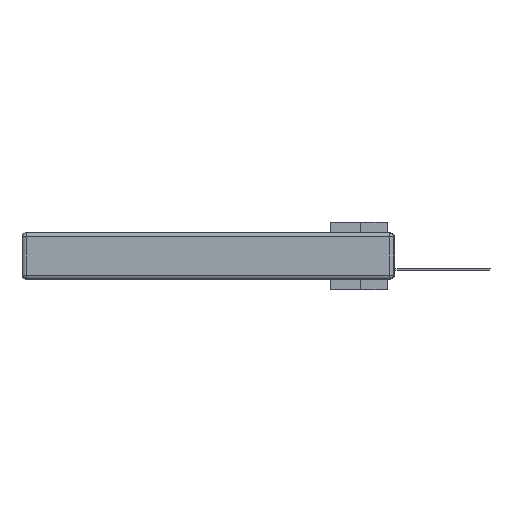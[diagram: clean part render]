
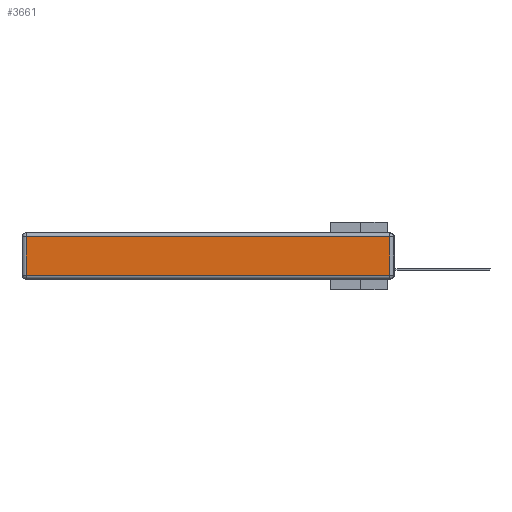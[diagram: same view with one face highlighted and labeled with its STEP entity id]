
A CAD part, left-side view. The second image highlights one B-rep face of the part: STEP entity #3661.
In plain terms, the highlighted planar face has unit normal (-1, 0, 0).
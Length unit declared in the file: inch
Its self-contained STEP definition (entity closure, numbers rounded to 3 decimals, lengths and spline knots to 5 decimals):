
#362 = CARTESIAN_POINT ( 'NONE',  ( 0., 0., -0.343 ) ) ;
#374 = EDGE_CURVE ( 'NONE', #20230, #2573, #5183, .T. ) ;
#2291 = VERTEX_POINT ( 'NONE', #15961 ) ;
#2573 = VERTEX_POINT ( 'NONE', #19842 ) ;
#3267 = DIRECTION ( 'NONE',  ( 0., -1., 0. ) ) ;
#3422 = CARTESIAN_POINT ( 'NONE',  ( 0., 0.03, -0.343 ) ) ;
#3661 = ADVANCED_FACE ( 'NONE', ( #16347 ), #23133, .T. ) ;
#4164 = VERTEX_POINT ( 'NONE', #18203 ) ;
#4751 = ORIENTED_EDGE ( 'NONE', *, *, #374, .T. ) ;
#5183 = LINE ( 'NONE', #23361, #8716 ) ;
#6551 = LINE ( 'NONE', #23676, #21385 ) ;
#7137 = EDGE_LOOP ( 'NONE', ( #4751, #26749, #14379, #14037 ) ) ;
#7951 = DIRECTION ( 'NONE',  ( 0., 0., 1. ) ) ;
#8066 = VECTOR ( 'NONE', #22268, 39.37008 ) ;
#8716 = VECTOR ( 'NONE', #3267, 39.37008 ) ;
#9574 = DIRECTION ( 'NONE',  ( -1., 0., 0. ) ) ;
#11588 = DIRECTION ( 'NONE',  ( 0., 0., 1. ) ) ;
#13783 = LINE ( 'NONE', #17751, #8066 ) ;
#14037 = ORIENTED_EDGE ( 'NONE', *, *, #17062, .T. ) ;
#14379 = ORIENTED_EDGE ( 'NONE', *, *, #21149, .T. ) ;
#15961 = CARTESIAN_POINT ( 'NONE',  ( 0., 0.03, -0.03 ) ) ;
#16347 = FACE_OUTER_BOUND ( 'NONE', #7137, .T. ) ;
#16364 = EDGE_CURVE ( 'NONE', #2573, #2291, #17920, .T. ) ;
#17062 = EDGE_CURVE ( 'NONE', #4164, #20230, #6551, .T. ) ;
#17751 = CARTESIAN_POINT ( 'NONE',  ( 0., 2.75, -0.03 ) ) ;
#17920 = LINE ( 'NONE', #3422, #25281 ) ;
#18203 = CARTESIAN_POINT ( 'NONE',  ( 0., 2.72, -0.03 ) ) ;
#19842 = CARTESIAN_POINT ( 'NONE',  ( 0., 0.03, -0.313 ) ) ;
#20230 = VERTEX_POINT ( 'NONE', #27664 ) ;
#21149 = EDGE_CURVE ( 'NONE', #2291, #4164, #13783, .T. ) ;
#21385 = VECTOR ( 'NONE', #21522, 39.37008 ) ;
#21522 = DIRECTION ( 'NONE',  ( 0., 0., -1. ) ) ;
#22268 = DIRECTION ( 'NONE',  ( 0., 1., 0. ) ) ;
#23133 = PLANE ( 'NONE',  #25369 ) ;
#23361 = CARTESIAN_POINT ( 'NONE',  ( 0., 0., -0.313 ) ) ;
#23676 = CARTESIAN_POINT ( 'NONE',  ( 0., 2.72, -0.343 ) ) ;
#25281 = VECTOR ( 'NONE', #7951, 39.37008 ) ;
#25369 = AXIS2_PLACEMENT_3D ( 'NONE', #362, #9574, #11588 ) ;
#26749 = ORIENTED_EDGE ( 'NONE', *, *, #16364, .T. ) ;
#27664 = CARTESIAN_POINT ( 'NONE',  ( 0., 2.72, -0.313 ) ) ;
